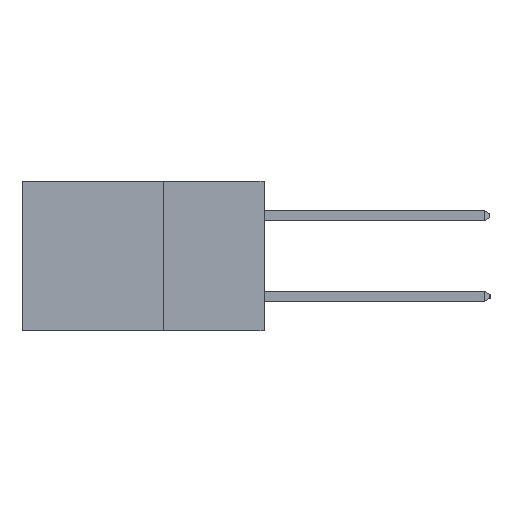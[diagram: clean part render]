
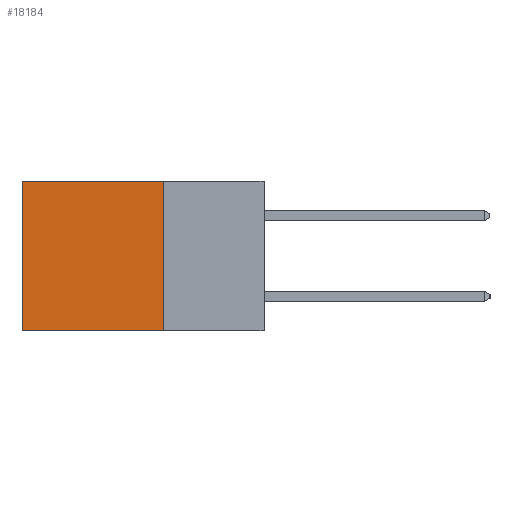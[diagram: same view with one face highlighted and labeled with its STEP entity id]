
A CAD part, left-side view. The second image highlights one B-rep face of the part: STEP entity #18184.
In plain terms, the highlighted planar face has unit normal (-1, 0, 0).
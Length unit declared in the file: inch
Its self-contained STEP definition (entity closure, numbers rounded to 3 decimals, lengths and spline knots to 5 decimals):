
#237 = VECTOR ( 'NONE', #11883, 39.37008 ) ;
#1364 = LINE ( 'NONE', #4947, #12349 ) ;
#2513 = LINE ( 'NONE', #21693, #17395 ) ;
#3562 = AXIS2_PLACEMENT_3D ( 'NONE', #19258, #21167, #9675 ) ;
#3781 = ORIENTED_EDGE ( 'NONE', *, *, #8128, .T. ) ;
#4794 = EDGE_CURVE ( 'NONE', #9670, #14442, #9216, .T. ) ;
#4947 = CARTESIAN_POINT ( 'NONE',  ( 0.2615, 0.6, -0.37 ) ) ;
#5729 = PLANE ( 'NONE',  #3562 ) ;
#8128 = EDGE_CURVE ( 'NONE', #8723, #8888, #1364, .T. ) ;
#8238 = DIRECTION ( 'NONE',  ( 0., 1., 0. ) ) ;
#8334 = EDGE_LOOP ( 'NONE', ( #3781, #19185, #10336, #18149 ) ) ;
#8723 = VERTEX_POINT ( 'NONE', #12579 ) ;
#8888 = VERTEX_POINT ( 'NONE', #18730 ) ;
#9216 = LINE ( 'NONE', #10775, #14352 ) ;
#9670 = VERTEX_POINT ( 'NONE', #23022 ) ;
#9675 = DIRECTION ( 'NONE',  ( 0., 0., -1. ) ) ;
#9943 = CARTESIAN_POINT ( 'NONE',  ( 0.2615, 0.25, -0.37 ) ) ;
#10336 = ORIENTED_EDGE ( 'NONE', *, *, #4794, .F. ) ;
#10775 = CARTESIAN_POINT ( 'NONE',  ( 0.2615, 0.25, -0.37 ) ) ;
#11883 = DIRECTION ( 'NONE',  ( 0., 1., 0. ) ) ;
#12349 = VECTOR ( 'NONE', #18515, 39.37008 ) ;
#12414 = CARTESIAN_POINT ( 'NONE',  ( 0.2615, 0.25, -0.37 ) ) ;
#12579 = CARTESIAN_POINT ( 'NONE',  ( 0.2615, 0.6, 0. ) ) ;
#14352 = VECTOR ( 'NONE', #24135, 39.37008 ) ;
#14442 = VERTEX_POINT ( 'NONE', #12414 ) ;
#15818 = LINE ( 'NONE', #9943, #237 ) ;
#17395 = VECTOR ( 'NONE', #8238, 39.37008 ) ;
#18149 = ORIENTED_EDGE ( 'NONE', *, *, #22087, .T. ) ;
#18184 = ADVANCED_FACE ( 'NONE', ( #18461 ), #5729, .F. ) ;
#18461 = FACE_OUTER_BOUND ( 'NONE', #8334, .T. ) ;
#18515 = DIRECTION ( 'NONE',  ( 0., 0., -1. ) ) ;
#18730 = CARTESIAN_POINT ( 'NONE',  ( 0.2615, 0.6, -0.37 ) ) ;
#19185 = ORIENTED_EDGE ( 'NONE', *, *, #23655, .F. ) ;
#19258 = CARTESIAN_POINT ( 'NONE',  ( 0.2615, 0.25, -0.37 ) ) ;
#21167 = DIRECTION ( 'NONE',  ( 1., 0., 0. ) ) ;
#21693 = CARTESIAN_POINT ( 'NONE',  ( 0.2615, 0.25, 0. ) ) ;
#22087 = EDGE_CURVE ( 'NONE', #9670, #8723, #2513, .T. ) ;
#23022 = CARTESIAN_POINT ( 'NONE',  ( 0.2615, 0.25, 0. ) ) ;
#23655 = EDGE_CURVE ( 'NONE', #14442, #8888, #15818, .T. ) ;
#24135 = DIRECTION ( 'NONE',  ( 0., 0., -1. ) ) ;
